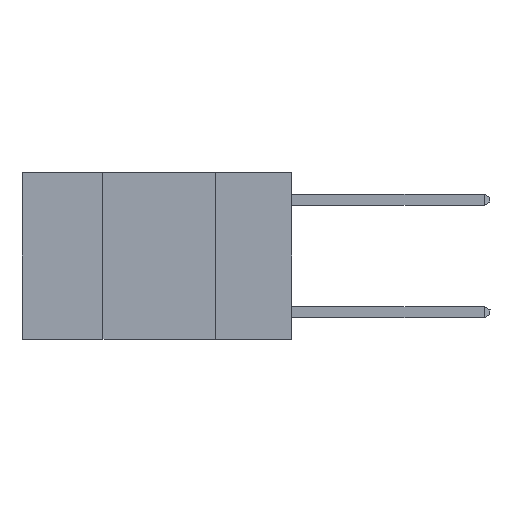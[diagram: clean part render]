
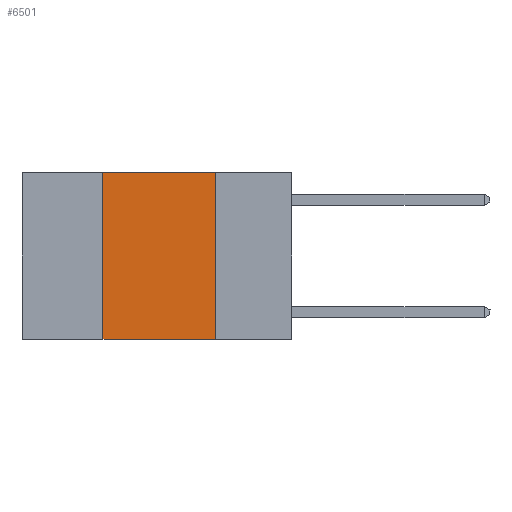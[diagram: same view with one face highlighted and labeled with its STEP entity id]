
A CAD part, left-side view. The second image highlights one B-rep face of the part: STEP entity #6501.
In plain terms, the highlighted planar face has unit normal (-1, 0, 0).
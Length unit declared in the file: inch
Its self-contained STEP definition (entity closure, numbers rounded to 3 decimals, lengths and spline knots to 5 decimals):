
#3 = VERTEX_POINT ( 'NONE', #17169 ) ;
#48 = CARTESIAN_POINT ( 'NONE',  ( 0., 0.6, 0. ) ) ;
#119 = FACE_OUTER_BOUND ( 'NONE', #1268, .T. ) ;
#347 = ORIENTED_EDGE ( 'NONE', *, *, #13114, .F. ) ;
#1268 = EDGE_LOOP ( 'NONE', ( #347, #13561, #5647, #8073 ) ) ;
#1510 = VERTEX_POINT ( 'NONE', #8137 ) ;
#1617 = AXIS2_PLACEMENT_3D ( 'NONE', #17235, #3691, #13296 ) ;
#1897 = VECTOR ( 'NONE', #5639, 39.37008 ) ;
#2233 = VECTOR ( 'NONE', #3753, 39.37008 ) ;
#2709 = LINE ( 'NONE', #48, #13250 ) ;
#3691 = DIRECTION ( 'NONE',  ( 1., 0., 0. ) ) ;
#3711 = DIRECTION ( 'NONE',  ( 0., -1., 0. ) ) ;
#3753 = DIRECTION ( 'NONE',  ( 0., 0., 1. ) ) ;
#4253 = CARTESIAN_POINT ( 'NONE',  ( 0., 0.17, 0. ) ) ;
#5639 = DIRECTION ( 'NONE',  ( 0., 0., -1. ) ) ;
#5647 = ORIENTED_EDGE ( 'NONE', *, *, #15706, .F. ) ;
#5781 = EDGE_CURVE ( 'NONE', #1510, #11419, #11052, .T. ) ;
#5852 = CARTESIAN_POINT ( 'NONE',  ( 0., 0.17, -0.37 ) ) ;
#6501 = ADVANCED_FACE ( 'NONE', ( #119 ), #11925, .F. ) ;
#7031 = DIRECTION ( 'NONE',  ( 0., -1., 0. ) ) ;
#8073 = ORIENTED_EDGE ( 'NONE', *, *, #5781, .T. ) ;
#8137 = CARTESIAN_POINT ( 'NONE',  ( 0., 0.42, -0.37 ) ) ;
#8784 = VERTEX_POINT ( 'NONE', #12483 ) ;
#9297 = LINE ( 'NONE', #4253, #1897 ) ;
#11052 = LINE ( 'NONE', #13259, #17720 ) ;
#11419 = VERTEX_POINT ( 'NONE', #5852 ) ;
#11925 = PLANE ( 'NONE',  #1617 ) ;
#12483 = CARTESIAN_POINT ( 'NONE',  ( 0., 0.42, 0. ) ) ;
#13114 = EDGE_CURVE ( 'NONE', #3, #11419, #9297, .T. ) ;
#13250 = VECTOR ( 'NONE', #7031, 39.37008 ) ;
#13259 = CARTESIAN_POINT ( 'NONE',  ( 0., 0.6, -0.37 ) ) ;
#13296 = DIRECTION ( 'NONE',  ( 0., 0., -1. ) ) ;
#13354 = CARTESIAN_POINT ( 'NONE',  ( 0., 0.42, 0. ) ) ;
#13561 = ORIENTED_EDGE ( 'NONE', *, *, #14778, .F. ) ;
#13641 = LINE ( 'NONE', #13354, #2233 ) ;
#14778 = EDGE_CURVE ( 'NONE', #8784, #3, #2709, .T. ) ;
#15706 = EDGE_CURVE ( 'NONE', #1510, #8784, #13641, .T. ) ;
#17169 = CARTESIAN_POINT ( 'NONE',  ( 0., 0.17, 0. ) ) ;
#17235 = CARTESIAN_POINT ( 'NONE',  ( 0., 0.6, 0. ) ) ;
#17720 = VECTOR ( 'NONE', #3711, 39.37008 ) ;
